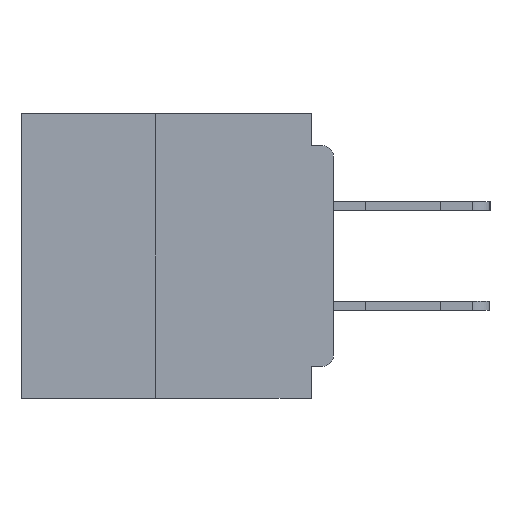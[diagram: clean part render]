
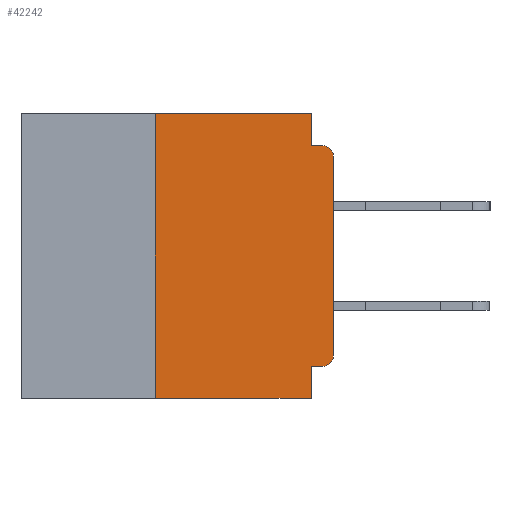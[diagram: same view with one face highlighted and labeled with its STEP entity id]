
A CAD part, left-side view. The second image highlights one B-rep face of the part: STEP entity #42242.
In plain terms, the highlighted planar face has unit normal (-1, 0, 0).
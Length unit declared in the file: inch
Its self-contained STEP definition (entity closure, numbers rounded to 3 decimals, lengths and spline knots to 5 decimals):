
#162 = PLANE ( 'NONE',  #5802 ) ;
#308 = DIRECTION ( 'NONE',  ( 1., 0., 0. ) ) ;
#1307 = DIRECTION ( 'NONE',  ( -1., 0., 0. ) ) ;
#1598 = DIRECTION ( 'NONE',  ( 0., -1., 0. ) ) ;
#1695 = ORIENTED_EDGE ( 'NONE', *, *, #18861, .F. ) ;
#2810 = EDGE_CURVE ( 'NONE', #18206, #41767, #30283, .T. ) ;
#3599 = VECTOR ( 'NONE', #18890, 39.37008 ) ;
#4057 = CARTESIAN_POINT ( 'NONE',  ( 0., 0.031, -0.4 ) ) ;
#4782 = DIRECTION ( 'NONE',  ( 0., 0., -1. ) ) ;
#5021 = DIRECTION ( 'NONE',  ( 0., -1., 0. ) ) ;
#5584 = DIRECTION ( 'NONE',  ( 0., 0., 1. ) ) ;
#5598 = EDGE_CURVE ( 'NONE', #41767, #18739, #7967, .T. ) ;
#5802 = AXIS2_PLACEMENT_3D ( 'NONE', #32860, #308, #23100 ) ;
#6394 = ORIENTED_EDGE ( 'NONE', *, *, #26048, .T. ) ;
#7684 = DIRECTION ( 'NONE',  ( -1., 0., 0. ) ) ;
#7967 = LINE ( 'NONE', #24408, #32944 ) ;
#8190 = VERTEX_POINT ( 'NONE', #4057 ) ;
#8236 = EDGE_CURVE ( 'NONE', #21189, #40134, #26033, .T. ) ;
#8400 = FACE_OUTER_BOUND ( 'NONE', #21759, .T. ) ;
#10508 = LINE ( 'NONE', #21023, #18081 ) ;
#10836 = VECTOR ( 'NONE', #23030, 39.37008 ) ;
#10905 = ORIENTED_EDGE ( 'NONE', *, *, #16746, .F. ) ;
#11735 = DIRECTION ( 'NONE',  ( 0., -1., 0. ) ) ;
#12395 = CARTESIAN_POINT ( 'NONE',  ( 0., 0., -0.355 ) ) ;
#12745 = VERTEX_POINT ( 'NONE', #25768 ) ;
#13606 = VERTEX_POINT ( 'NONE', #40304 ) ;
#13840 = EDGE_CURVE ( 'NONE', #36221, #13606, #19553, .T. ) ;
#15078 = ORIENTED_EDGE ( 'NONE', *, *, #2810, .F. ) ;
#15245 = ORIENTED_EDGE ( 'NONE', *, *, #37024, .F. ) ;
#15822 = CARTESIAN_POINT ( 'NONE',  ( 0., 0.25, -0.4 ) ) ;
#16746 = EDGE_CURVE ( 'NONE', #40340, #8190, #10508, .T. ) ;
#17636 = ORIENTED_EDGE ( 'NONE', *, *, #13840, .T. ) ;
#18081 = VECTOR ( 'NONE', #4782, 39.37008 ) ;
#18109 = EDGE_CURVE ( 'NONE', #18739, #12745, #33315, .T. ) ;
#18206 = VERTEX_POINT ( 'NONE', #15822 ) ;
#18739 = VERTEX_POINT ( 'NONE', #21455 ) ;
#18861 = EDGE_CURVE ( 'NONE', #21189, #40340, #29689, .T. ) ;
#18890 = DIRECTION ( 'NONE',  ( 0., 1., 0. ) ) ;
#19437 = LINE ( 'NONE', #39356, #10836 ) ;
#19553 = CIRCLE ( 'NONE', #34283, 0.015 ) ;
#20590 = CARTESIAN_POINT ( 'NONE',  ( 0., 0.25, 0. ) ) ;
#20824 = CARTESIAN_POINT ( 'NONE',  ( 0., 0.015, -0.06 ) ) ;
#21023 = CARTESIAN_POINT ( 'NONE',  ( 0., 0.031, -0.4 ) ) ;
#21189 = VERTEX_POINT ( 'NONE', #22031 ) ;
#21264 = CARTESIAN_POINT ( 'NONE',  ( 0., 0., -0.045 ) ) ;
#21455 = CARTESIAN_POINT ( 'NONE',  ( 0., 0.031, 0. ) ) ;
#21522 = VECTOR ( 'NONE', #5584, 39.37008 ) ;
#21759 = EDGE_LOOP ( 'NONE', ( #6394, #17636, #15245, #25947, #35146, #15078, #22689, #10905, #1695, #35289 ) ) ;
#22031 = CARTESIAN_POINT ( 'NONE',  ( 0., 0.015, -0.355 ) ) ;
#22689 = ORIENTED_EDGE ( 'NONE', *, *, #27703, .T. ) ;
#23030 = DIRECTION ( 'NONE',  ( 0., 0., 1. ) ) ;
#23100 = DIRECTION ( 'NONE',  ( 0., 0., -1. ) ) ;
#23160 = CARTESIAN_POINT ( 'NONE',  ( 0., 0., -0.06 ) ) ;
#23540 = VECTOR ( 'NONE', #38113, 39.37008 ) ;
#24090 = DIRECTION ( 'NONE',  ( 0., 0., -1. ) ) ;
#24240 = VECTOR ( 'NONE', #5021, 39.37008 ) ;
#24408 = CARTESIAN_POINT ( 'NONE',  ( 0., 0.437, 0. ) ) ;
#24957 = CARTESIAN_POINT ( 'NONE',  ( 0., 0.25, -0.4 ) ) ;
#25768 = CARTESIAN_POINT ( 'NONE',  ( 0., 0.031, -0.045 ) ) ;
#25947 = ORIENTED_EDGE ( 'NONE', *, *, #18109, .F. ) ;
#26033 = CIRCLE ( 'NONE', #39096, 0.015 ) ;
#26048 = EDGE_CURVE ( 'NONE', #40134, #36221, #19437, .T. ) ;
#27196 = CARTESIAN_POINT ( 'NONE',  ( 0., 0.015, -0.34 ) ) ;
#27490 = LINE ( 'NONE', #34536, #34157 ) ;
#27703 = EDGE_CURVE ( 'NONE', #18206, #8190, #27490, .T. ) ;
#29689 = LINE ( 'NONE', #12395, #3599 ) ;
#30283 = LINE ( 'NONE', #24957, #21522 ) ;
#30508 = DIRECTION ( 'NONE',  ( 0., 0., -1. ) ) ;
#31528 = CARTESIAN_POINT ( 'NONE',  ( 0., 0.031, 0. ) ) ;
#32860 = CARTESIAN_POINT ( 'NONE',  ( 0., 0.437, 0. ) ) ;
#32944 = VECTOR ( 'NONE', #1598, 39.37008 ) ;
#33315 = LINE ( 'NONE', #31528, #23540 ) ;
#34028 = LINE ( 'NONE', #21264, #24240 ) ;
#34157 = VECTOR ( 'NONE', #11735, 39.37008 ) ;
#34283 = AXIS2_PLACEMENT_3D ( 'NONE', #20824, #1307, #24090 ) ;
#34536 = CARTESIAN_POINT ( 'NONE',  ( 0., 0.437, -0.4 ) ) ;
#35065 = CARTESIAN_POINT ( 'NONE',  ( 0., 0., -0.34 ) ) ;
#35146 = ORIENTED_EDGE ( 'NONE', *, *, #5598, .F. ) ;
#35289 = ORIENTED_EDGE ( 'NONE', *, *, #8236, .T. ) ;
#36187 = CARTESIAN_POINT ( 'NONE',  ( 0., 0.031, -0.355 ) ) ;
#36221 = VERTEX_POINT ( 'NONE', #23160 ) ;
#37024 = EDGE_CURVE ( 'NONE', #12745, #13606, #34028, .T. ) ;
#38113 = DIRECTION ( 'NONE',  ( 0., 0., -1. ) ) ;
#39096 = AXIS2_PLACEMENT_3D ( 'NONE', #27196, #7684, #30508 ) ;
#39356 = CARTESIAN_POINT ( 'NONE',  ( 0., 0., 0. ) ) ;
#40134 = VERTEX_POINT ( 'NONE', #35065 ) ;
#40304 = CARTESIAN_POINT ( 'NONE',  ( 0., 0.015, -0.045 ) ) ;
#40340 = VERTEX_POINT ( 'NONE', #36187 ) ;
#41767 = VERTEX_POINT ( 'NONE', #20590 ) ;
#42242 = ADVANCED_FACE ( 'NONE', ( #8400 ), #162, .F. ) ;
